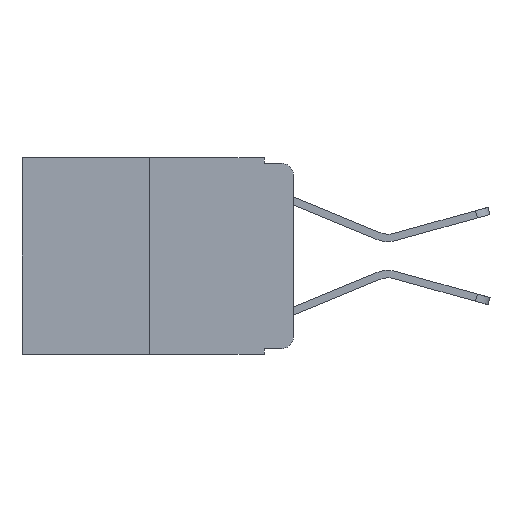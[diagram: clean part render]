
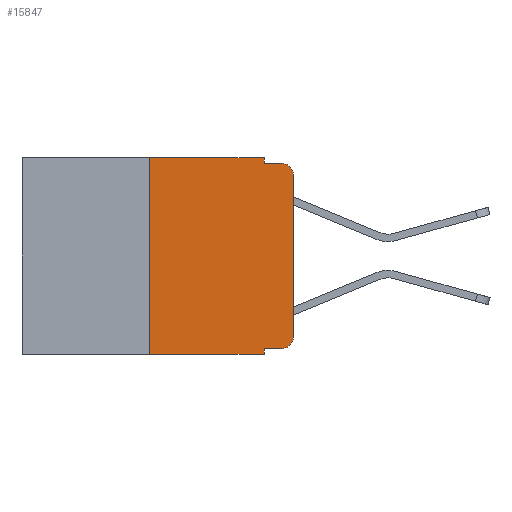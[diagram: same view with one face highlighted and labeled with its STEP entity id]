
A CAD part, left-side view. The second image highlights one B-rep face of the part: STEP entity #15847.
In plain terms, the highlighted planar face has unit normal (-1, 0, 0).
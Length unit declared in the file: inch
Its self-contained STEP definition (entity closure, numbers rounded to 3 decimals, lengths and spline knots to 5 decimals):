
#815 = LINE ( 'NONE', #13275, #21455 ) ;
#967 = LINE ( 'NONE', #3216, #9287 ) ;
#1091 = ORIENTED_EDGE ( 'NONE', *, *, #7212, .T. ) ;
#1403 = VERTEX_POINT ( 'NONE', #15211 ) ;
#1470 = LINE ( 'NONE', #9353, #1794 ) ;
#1521 = DIRECTION ( 'NONE',  ( 0., 0., 1. ) ) ;
#1668 = DIRECTION ( 'NONE',  ( 0., 0., -1. ) ) ;
#1794 = VECTOR ( 'NONE', #15564, 39.37008 ) ;
#2876 = DIRECTION ( 'NONE',  ( 0., 0., -1. ) ) ;
#2882 = AXIS2_PLACEMENT_3D ( 'NONE', #6884, #23156, #8945 ) ;
#3179 = CIRCLE ( 'NONE', #13637, 0.02 ) ;
#3216 = CARTESIAN_POINT ( 'NONE',  ( 0., 0.473, 0. ) ) ;
#3936 = CARTESIAN_POINT ( 'NONE',  ( 0., 0.051, -0.333 ) ) ;
#4090 = CARTESIAN_POINT ( 'NONE',  ( 0., 0., -0.313 ) ) ;
#5073 = VERTEX_POINT ( 'NONE', #4090 ) ;
#5272 = EDGE_CURVE ( 'NONE', #10345, #18508, #10832, .T. ) ;
#5885 = VECTOR ( 'NONE', #7239, 39.37008 ) ;
#6283 = ORIENTED_EDGE ( 'NONE', *, *, #23817, .T. ) ;
#6286 = EDGE_CURVE ( 'NONE', #11530, #11609, #22727, .T. ) ;
#6748 = EDGE_CURVE ( 'NONE', #11609, #26354, #17602, .T. ) ;
#6884 = CARTESIAN_POINT ( 'NONE',  ( 0., 0.473, 0. ) ) ;
#7212 = EDGE_CURVE ( 'NONE', #5073, #25128, #7395, .T. ) ;
#7239 = DIRECTION ( 'NONE',  ( 0., 0., -1. ) ) ;
#7308 = VECTOR ( 'NONE', #17973, 39.37008 ) ;
#7395 = LINE ( 'NONE', #19564, #18224 ) ;
#8910 = CIRCLE ( 'NONE', #16133, 0.02 ) ;
#8945 = DIRECTION ( 'NONE',  ( 0., 0., -1. ) ) ;
#9287 = VECTOR ( 'NONE', #13451, 39.37008 ) ;
#9353 = CARTESIAN_POINT ( 'NONE',  ( 0., 0.25, 0. ) ) ;
#9435 = CARTESIAN_POINT ( 'NONE',  ( 0., 0.051, 0. ) ) ;
#9576 = FACE_OUTER_BOUND ( 'NONE', #26174, .T. ) ;
#9644 = DIRECTION ( 'NONE',  ( 0., 0., -1. ) ) ;
#9829 = EDGE_CURVE ( 'NONE', #25128, #26354, #8910, .T. ) ;
#10345 = VERTEX_POINT ( 'NONE', #14884 ) ;
#10647 = ORIENTED_EDGE ( 'NONE', *, *, #6748, .F. ) ;
#10832 = LINE ( 'NONE', #3936, #7308 ) ;
#10959 = CARTESIAN_POINT ( 'NONE',  ( 0., 0.02, -0.313 ) ) ;
#11325 = CARTESIAN_POINT ( 'NONE',  ( 0., 0.02, -0.01 ) ) ;
#11530 = VERTEX_POINT ( 'NONE', #9435 ) ;
#11609 = VERTEX_POINT ( 'NONE', #13788 ) ;
#11692 = EDGE_CURVE ( 'NONE', #24009, #11530, #967, .T. ) ;
#11857 = ORIENTED_EDGE ( 'NONE', *, *, #25769, .F. ) ;
#11911 = VECTOR ( 'NONE', #23282, 39.37008 ) ;
#11993 = EDGE_CURVE ( 'NONE', #10345, #18682, #21473, .T. ) ;
#13275 = CARTESIAN_POINT ( 'NONE',  ( 0., 0.473, -0.343 ) ) ;
#13451 = DIRECTION ( 'NONE',  ( 0., -1., 0. ) ) ;
#13637 = AXIS2_PLACEMENT_3D ( 'NONE', #10959, #22948, #2876 ) ;
#13652 = ORIENTED_EDGE ( 'NONE', *, *, #9829, .T. ) ;
#13668 = CARTESIAN_POINT ( 'NONE',  ( 0., 0.02, -0.03 ) ) ;
#13788 = CARTESIAN_POINT ( 'NONE',  ( 0., 0.051, -0.01 ) ) ;
#14164 = ORIENTED_EDGE ( 'NONE', *, *, #16354, .T. ) ;
#14587 = ORIENTED_EDGE ( 'NONE', *, *, #11692, .F. ) ;
#14884 = CARTESIAN_POINT ( 'NONE',  ( 0., 0.051, -0.333 ) ) ;
#15211 = CARTESIAN_POINT ( 'NONE',  ( 0., 0.25, -0.343 ) ) ;
#15564 = DIRECTION ( 'NONE',  ( 0., 0., 1. ) ) ;
#15642 = CARTESIAN_POINT ( 'NONE',  ( 0., 0.25, 0. ) ) ;
#15847 = ADVANCED_FACE ( 'NONE', ( #9576 ), #17091, .F. ) ;
#16133 = AXIS2_PLACEMENT_3D ( 'NONE', #13668, #17727, #9644 ) ;
#16354 = EDGE_CURVE ( 'NONE', #18508, #5073, #3179, .T. ) ;
#17091 = PLANE ( 'NONE',  #2882 ) ;
#17239 = DIRECTION ( 'NONE',  ( 0., -1., 0. ) ) ;
#17602 = LINE ( 'NONE', #25621, #11911 ) ;
#17727 = DIRECTION ( 'NONE',  ( -1., 0., 0. ) ) ;
#17973 = DIRECTION ( 'NONE',  ( 0., -1., 0. ) ) ;
#18224 = VECTOR ( 'NONE', #1521, 39.37008 ) ;
#18508 = VERTEX_POINT ( 'NONE', #19858 ) ;
#18682 = VERTEX_POINT ( 'NONE', #20638 ) ;
#19410 = CARTESIAN_POINT ( 'NONE',  ( 0., 0.051, 0. ) ) ;
#19449 = ORIENTED_EDGE ( 'NONE', *, *, #5272, .T. ) ;
#19564 = CARTESIAN_POINT ( 'NONE',  ( 0., 0., 0. ) ) ;
#19858 = CARTESIAN_POINT ( 'NONE',  ( 0., 0.02, -0.333 ) ) ;
#20638 = CARTESIAN_POINT ( 'NONE',  ( 0., 0.051, -0.343 ) ) ;
#20853 = VECTOR ( 'NONE', #1668, 39.37008 ) ;
#21455 = VECTOR ( 'NONE', #17239, 39.37008 ) ;
#21473 = LINE ( 'NONE', #23916, #20853 ) ;
#22727 = LINE ( 'NONE', #19410, #5885 ) ;
#22948 = DIRECTION ( 'NONE',  ( -1., 0., 0. ) ) ;
#23156 = DIRECTION ( 'NONE',  ( 1., 0., 0. ) ) ;
#23166 = ORIENTED_EDGE ( 'NONE', *, *, #11993, .F. ) ;
#23282 = DIRECTION ( 'NONE',  ( 0., -1., 0. ) ) ;
#23817 = EDGE_CURVE ( 'NONE', #1403, #18682, #815, .T. ) ;
#23916 = CARTESIAN_POINT ( 'NONE',  ( 0., 0.051, 0. ) ) ;
#24009 = VERTEX_POINT ( 'NONE', #15642 ) ;
#25128 = VERTEX_POINT ( 'NONE', #25491 ) ;
#25165 = ORIENTED_EDGE ( 'NONE', *, *, #6286, .F. ) ;
#25491 = CARTESIAN_POINT ( 'NONE',  ( 0., 0., -0.03 ) ) ;
#25621 = CARTESIAN_POINT ( 'NONE',  ( 0., 0.051, -0.01 ) ) ;
#25769 = EDGE_CURVE ( 'NONE', #1403, #24009, #1470, .T. ) ;
#26174 = EDGE_LOOP ( 'NONE', ( #1091, #13652, #10647, #25165, #14587, #11857, #6283, #23166, #19449, #14164 ) ) ;
#26354 = VERTEX_POINT ( 'NONE', #11325 ) ;
